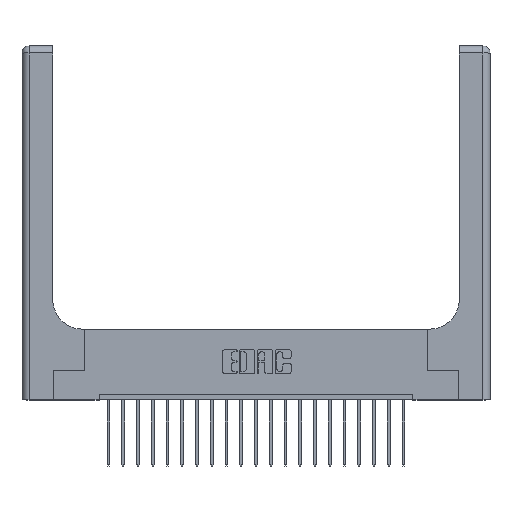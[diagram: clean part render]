
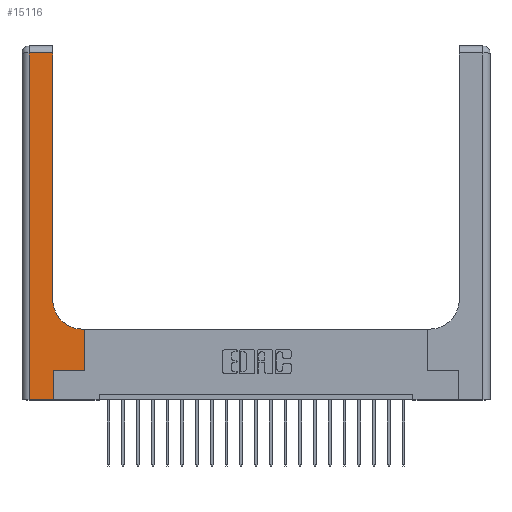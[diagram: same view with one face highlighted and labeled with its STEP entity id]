
A CAD part, top view. The second image highlights one B-rep face of the part: STEP entity #15116.
In plain terms, the highlighted planar face has unit normal (0, 0, 1).
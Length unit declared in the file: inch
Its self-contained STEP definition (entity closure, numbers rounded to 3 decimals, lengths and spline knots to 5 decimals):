
#20 = VECTOR ( 'NONE', #18074, 39.37008 ) ;
#278 = DIRECTION ( 'NONE',  ( 0., 0., -1. ) ) ;
#486 = EDGE_CURVE ( 'NONE', #13890, #10579, #19973, .T. ) ;
#494 = LINE ( 'NONE', #15736, #13014 ) ;
#676 = EDGE_CURVE ( 'NONE', #10579, #20324, #7753, .T. ) ;
#1008 = CARTESIAN_POINT ( 'NONE',  ( 0.06, 0., 0.37 ) ) ;
#1618 = EDGE_LOOP ( 'NONE', ( #18595, #4840, #17757, #6121, #20254, #13263, #9349, #14026, #7573 ) ) ;
#1632 = LINE ( 'NONE', #11038, #17203 ) ;
#2657 = FACE_OUTER_BOUND ( 'NONE', #1618, .T. ) ;
#3261 = EDGE_CURVE ( 'NONE', #3470, #18497, #4769, .T. ) ;
#3397 = VECTOR ( 'NONE', #3849, 39.37008 ) ;
#3470 = VERTEX_POINT ( 'NONE', #14841 ) ;
#3508 = DIRECTION ( 'NONE',  ( 0., 1., 0. ) ) ;
#3849 = DIRECTION ( 'NONE',  ( -1., 0., 0. ) ) ;
#3870 = EDGE_CURVE ( 'NONE', #14750, #13890, #16008, .T. ) ;
#4681 = DIRECTION ( 'NONE',  ( 1., 0., 0. ) ) ;
#4769 = LINE ( 'NONE', #18606, #8645 ) ;
#4840 = ORIENTED_EDGE ( 'NONE', *, *, #676, .T. ) ;
#5055 = DIRECTION ( 'NONE',  ( 1., 0., 0. ) ) ;
#5193 = CARTESIAN_POINT ( 'NONE',  ( 0.51, 0.85, 0.37 ) ) ;
#5947 = VECTOR ( 'NONE', #3508, 39.37008 ) ;
#6121 = ORIENTED_EDGE ( 'NONE', *, *, #11242, .T. ) ;
#7447 = EDGE_CURVE ( 'NONE', #18465, #14750, #15579, .T. ) ;
#7551 = CARTESIAN_POINT ( 'NONE',  ( 0.528, 0.25, 0.37 ) ) ;
#7573 = ORIENTED_EDGE ( 'NONE', *, *, #3870, .T. ) ;
#7753 = LINE ( 'NONE', #8754, #3397 ) ;
#8327 = EDGE_CURVE ( 'NONE', #18497, #17304, #494, .T. ) ;
#8457 = CARTESIAN_POINT ( 'NONE',  ( 0.265, 0.25, 0.37 ) ) ;
#8645 = VECTOR ( 'NONE', #15428, 39.37008 ) ;
#8754 = CARTESIAN_POINT ( 'NONE',  ( 0., 2.94, 0.37 ) ) ;
#9341 = AXIS2_PLACEMENT_3D ( 'NONE', #5193, #278, #5055 ) ;
#9349 = ORIENTED_EDGE ( 'NONE', *, *, #10036, .T. ) ;
#9526 = DIRECTION ( 'NONE',  ( 0., 0., -1. ) ) ;
#10036 = EDGE_CURVE ( 'NONE', #17304, #18465, #14234, .T. ) ;
#10579 = VERTEX_POINT ( 'NONE', #17402 ) ;
#10935 = DIRECTION ( 'NONE',  ( 1., 0., 0. ) ) ;
#11038 = CARTESIAN_POINT ( 'NONE',  ( 0., 0., 0.37 ) ) ;
#11222 = VERTEX_POINT ( 'NONE', #1008 ) ;
#11242 = EDGE_CURVE ( 'NONE', #11222, #3470, #1632, .T. ) ;
#11423 = CARTESIAN_POINT ( 'NONE',  ( 0., 3., 0.37 ) ) ;
#11543 = CARTESIAN_POINT ( 'NONE',  ( 0.51, 0.6, 0.37 ) ) ;
#11931 = DIRECTION ( 'NONE',  ( 0., -1., 0. ) ) ;
#12790 = DIRECTION ( 'NONE',  ( -1., 0., 0. ) ) ;
#12998 = CARTESIAN_POINT ( 'NONE',  ( 0.528, 0.25, 0.37 ) ) ;
#13014 = VECTOR ( 'NONE', #10935, 39.37008 ) ;
#13263 = ORIENTED_EDGE ( 'NONE', *, *, #8327, .T. ) ;
#13890 = VERTEX_POINT ( 'NONE', #18181 ) ;
#14026 = ORIENTED_EDGE ( 'NONE', *, *, #7447, .T. ) ;
#14234 = LINE ( 'NONE', #12998, #19558 ) ;
#14658 = PLANE ( 'NONE',  #19923 ) ;
#14750 = VERTEX_POINT ( 'NONE', #11543 ) ;
#14841 = CARTESIAN_POINT ( 'NONE',  ( 0.265, 0., 0.37 ) ) ;
#15020 = CARTESIAN_POINT ( 'NONE',  ( 0.06, 3., 0.37 ) ) ;
#15116 = ADVANCED_FACE ( 'NONE', ( #2657 ), #14658, .F. ) ;
#15149 = CARTESIAN_POINT ( 'NONE',  ( 0.26, 3., 0.37 ) ) ;
#15428 = DIRECTION ( 'NONE',  ( 0., 1., 0. ) ) ;
#15579 = LINE ( 'NONE', #17293, #20 ) ;
#15644 = VECTOR ( 'NONE', #11931, 39.37008 ) ;
#15736 = CARTESIAN_POINT ( 'NONE',  ( 0.265, 0.25, 0.37 ) ) ;
#16008 = CIRCLE ( 'NONE', #9341, 0.25 ) ;
#16539 = EDGE_CURVE ( 'NONE', #20324, #11222, #19444, .T. ) ;
#16553 = CARTESIAN_POINT ( 'NONE',  ( 0.06, 2.94, 0.37 ) ) ;
#17203 = VECTOR ( 'NONE', #4681, 39.37008 ) ;
#17293 = CARTESIAN_POINT ( 'NONE',  ( 0.26, 0.6, 0.37 ) ) ;
#17304 = VERTEX_POINT ( 'NONE', #7551 ) ;
#17402 = CARTESIAN_POINT ( 'NONE',  ( 0.26, 2.94, 0.37 ) ) ;
#17757 = ORIENTED_EDGE ( 'NONE', *, *, #16539, .T. ) ;
#18074 = DIRECTION ( 'NONE',  ( -1., 0., 0. ) ) ;
#18181 = CARTESIAN_POINT ( 'NONE',  ( 0.26, 0.85, 0.37 ) ) ;
#18183 = CARTESIAN_POINT ( 'NONE',  ( 0.528, 0.6, 0.37 ) ) ;
#18366 = DIRECTION ( 'NONE',  ( 0., 1., 0. ) ) ;
#18465 = VERTEX_POINT ( 'NONE', #18183 ) ;
#18497 = VERTEX_POINT ( 'NONE', #8457 ) ;
#18595 = ORIENTED_EDGE ( 'NONE', *, *, #486, .T. ) ;
#18606 = CARTESIAN_POINT ( 'NONE',  ( 0.265, 0., 0.37 ) ) ;
#19444 = LINE ( 'NONE', #15020, #15644 ) ;
#19558 = VECTOR ( 'NONE', #18366, 39.37008 ) ;
#19923 = AXIS2_PLACEMENT_3D ( 'NONE', #11423, #9526, #12790 ) ;
#19973 = LINE ( 'NONE', #15149, #5947 ) ;
#20254 = ORIENTED_EDGE ( 'NONE', *, *, #3261, .T. ) ;
#20324 = VERTEX_POINT ( 'NONE', #16553 ) ;
